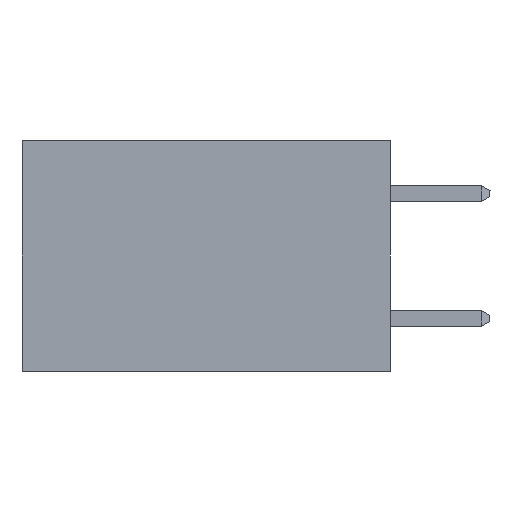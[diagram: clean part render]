
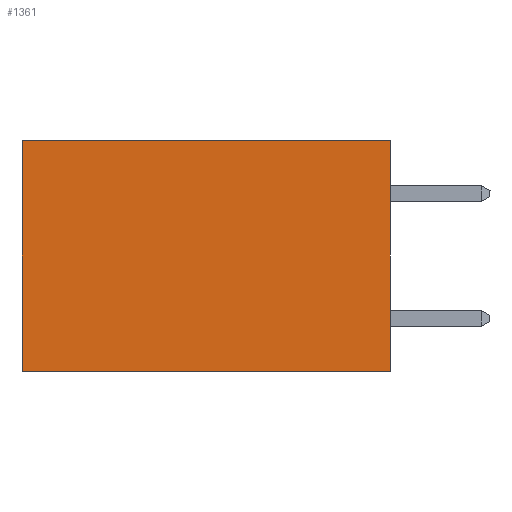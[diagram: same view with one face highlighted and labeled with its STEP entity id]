
A CAD part, left-side view. The second image highlights one B-rep face of the part: STEP entity #1361.
In plain terms, the highlighted planar face has unit normal (-1, 0, 0).
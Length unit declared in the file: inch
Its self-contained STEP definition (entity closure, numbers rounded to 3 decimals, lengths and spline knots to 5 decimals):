
#48 = EDGE_CURVE ( 'NONE', #4835, #7894, #3687, .T. ) ;
#73 = EDGE_CURVE ( 'NONE', #6682, #4835, #582, .T. ) ;
#582 = LINE ( 'NONE', #7433, #7803 ) ;
#972 = EDGE_LOOP ( 'NONE', ( #4078, #6376, #1740, #2076 ) ) ;
#1361 = ADVANCED_FACE ( 'NONE', ( #6233 ), #3901, .F. ) ;
#1740 = ORIENTED_EDGE ( 'NONE', *, *, #73, .F. ) ;
#2076 = ORIENTED_EDGE ( 'NONE', *, *, #4794, .T. ) ;
#3687 = LINE ( 'NONE', #9021, #8072 ) ;
#3901 = PLANE ( 'NONE',  #6468 ) ;
#4078 = ORIENTED_EDGE ( 'NONE', *, *, #11453, .T. ) ;
#4086 = VECTOR ( 'NONE', #9965, 39.37008 ) ;
#4141 = CARTESIAN_POINT ( 'NONE',  ( 0.277, 0., -0.37 ) ) ;
#4794 = EDGE_CURVE ( 'NONE', #6682, #11182, #6384, .T. ) ;
#4835 = VERTEX_POINT ( 'NONE', #4141 ) ;
#5215 = DIRECTION ( 'NONE',  ( 0., 0., -1. ) ) ;
#6233 = FACE_OUTER_BOUND ( 'NONE', #972, .T. ) ;
#6376 = ORIENTED_EDGE ( 'NONE', *, *, #48, .F. ) ;
#6384 = LINE ( 'NONE', #7388, #4086 ) ;
#6468 = AXIS2_PLACEMENT_3D ( 'NONE', #7722, #7782, #6823 ) ;
#6682 = VERTEX_POINT ( 'NONE', #8645 ) ;
#6823 = DIRECTION ( 'NONE',  ( 0., 0., -1. ) ) ;
#7388 = CARTESIAN_POINT ( 'NONE',  ( 0.277, 0., 0. ) ) ;
#7433 = CARTESIAN_POINT ( 'NONE',  ( 0.277, 0., -0.37 ) ) ;
#7722 = CARTESIAN_POINT ( 'NONE',  ( 0.277, 0., -0.37 ) ) ;
#7782 = DIRECTION ( 'NONE',  ( 1., 0., 0. ) ) ;
#7796 = CARTESIAN_POINT ( 'NONE',  ( 0.277, 0.59, -0.37 ) ) ;
#7803 = VECTOR ( 'NONE', #9300, 39.37008 ) ;
#7894 = VERTEX_POINT ( 'NONE', #10871 ) ;
#8072 = VECTOR ( 'NONE', #10927, 39.37008 ) ;
#8645 = CARTESIAN_POINT ( 'NONE',  ( 0.277, 0., 0. ) ) ;
#8751 = LINE ( 'NONE', #7796, #11442 ) ;
#9021 = CARTESIAN_POINT ( 'NONE',  ( 0.277, 0., -0.37 ) ) ;
#9300 = DIRECTION ( 'NONE',  ( 0., 0., -1. ) ) ;
#9965 = DIRECTION ( 'NONE',  ( 0., 1., 0. ) ) ;
#10871 = CARTESIAN_POINT ( 'NONE',  ( 0.277, 0.59, -0.37 ) ) ;
#10925 = CARTESIAN_POINT ( 'NONE',  ( 0.277, 0.59, 0. ) ) ;
#10927 = DIRECTION ( 'NONE',  ( 0., 1., 0. ) ) ;
#11182 = VERTEX_POINT ( 'NONE', #10925 ) ;
#11442 = VECTOR ( 'NONE', #5215, 39.37008 ) ;
#11453 = EDGE_CURVE ( 'NONE', #11182, #7894, #8751, .T. ) ;
